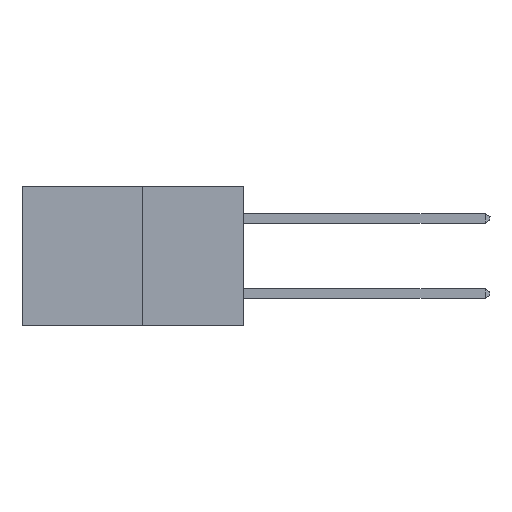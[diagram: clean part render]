
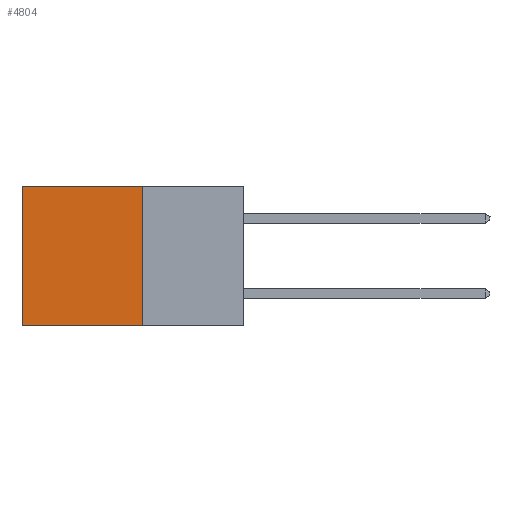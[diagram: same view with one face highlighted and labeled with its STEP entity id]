
A CAD part, left-side view. The second image highlights one B-rep face of the part: STEP entity #4804.
In plain terms, the highlighted planar face has unit normal (-1, 0, 0).
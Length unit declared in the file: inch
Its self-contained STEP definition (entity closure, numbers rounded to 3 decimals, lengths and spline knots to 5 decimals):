
#166 = VECTOR ( 'NONE', #1522, 39.37008 ) ;
#1225 = EDGE_CURVE ( 'NONE', #12703, #24298, #2958, .T. ) ;
#1334 = CARTESIAN_POINT ( 'NONE',  ( 0.277, 0.27, 0. ) ) ;
#1522 = DIRECTION ( 'NONE',  ( 0., 1., 0. ) ) ;
#2172 = EDGE_LOOP ( 'NONE', ( #6489, #5000, #17822, #5381 ) ) ;
#2958 = LINE ( 'NONE', #5394, #13085 ) ;
#3357 = AXIS2_PLACEMENT_3D ( 'NONE', #9808, #4153, #17412 ) ;
#4153 = DIRECTION ( 'NONE',  ( 1., 0., 0. ) ) ;
#4790 = DIRECTION ( 'NONE',  ( 0., 0., -1. ) ) ;
#4804 = ADVANCED_FACE ( 'NONE', ( #7862 ), #15527, .F. ) ;
#4847 = EDGE_CURVE ( 'NONE', #18492, #12703, #16740, .T. ) ;
#5000 = ORIENTED_EDGE ( 'NONE', *, *, #17302, .F. ) ;
#5381 = ORIENTED_EDGE ( 'NONE', *, *, #4847, .T. ) ;
#5394 = CARTESIAN_POINT ( 'NONE',  ( 0.277, 0.59, -0.37 ) ) ;
#6489 = ORIENTED_EDGE ( 'NONE', *, *, #1225, .T. ) ;
#7862 = FACE_OUTER_BOUND ( 'NONE', #2172, .T. ) ;
#8050 = DIRECTION ( 'NONE',  ( 0., 1., 0. ) ) ;
#9691 = VERTEX_POINT ( 'NONE', #18069 ) ;
#9808 = CARTESIAN_POINT ( 'NONE',  ( 0.277, 0.27, -0.37 ) ) ;
#10280 = CARTESIAN_POINT ( 'NONE',  ( 0.277, 0.59, 0. ) ) ;
#10348 = LINE ( 'NONE', #14758, #166 ) ;
#11056 = CARTESIAN_POINT ( 'NONE',  ( 0.277, 0.27, -0.37 ) ) ;
#12703 = VERTEX_POINT ( 'NONE', #10280 ) ;
#13085 = VECTOR ( 'NONE', #4790, 39.37008 ) ;
#14758 = CARTESIAN_POINT ( 'NONE',  ( 0.277, 0.27, -0.37 ) ) ;
#15527 = PLANE ( 'NONE',  #3357 ) ;
#16740 = LINE ( 'NONE', #19392, #21772 ) ;
#17302 = EDGE_CURVE ( 'NONE', #9691, #24298, #10348, .T. ) ;
#17412 = DIRECTION ( 'NONE',  ( 0., 0., -1. ) ) ;
#17424 = VECTOR ( 'NONE', #18677, 39.37008 ) ;
#17822 = ORIENTED_EDGE ( 'NONE', *, *, #17893, .F. ) ;
#17893 = EDGE_CURVE ( 'NONE', #18492, #9691, #22430, .T. ) ;
#18069 = CARTESIAN_POINT ( 'NONE',  ( 0.277, 0.27, -0.37 ) ) ;
#18492 = VERTEX_POINT ( 'NONE', #1334 ) ;
#18677 = DIRECTION ( 'NONE',  ( 0., 0., -1. ) ) ;
#19392 = CARTESIAN_POINT ( 'NONE',  ( 0.277, 0.27, 0. ) ) ;
#20508 = CARTESIAN_POINT ( 'NONE',  ( 0.277, 0.59, -0.37 ) ) ;
#21772 = VECTOR ( 'NONE', #8050, 39.37008 ) ;
#22430 = LINE ( 'NONE', #11056, #17424 ) ;
#24298 = VERTEX_POINT ( 'NONE', #20508 ) ;
